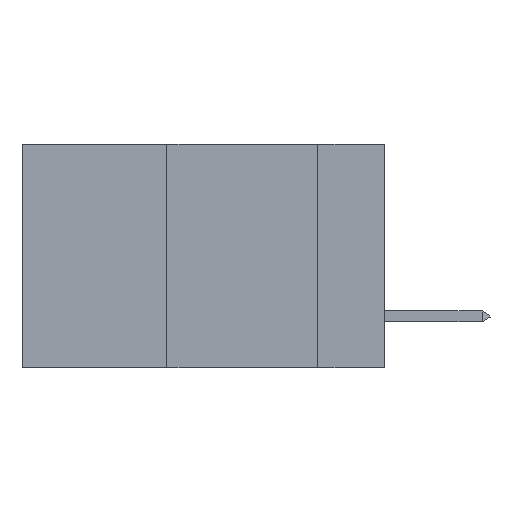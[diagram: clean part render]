
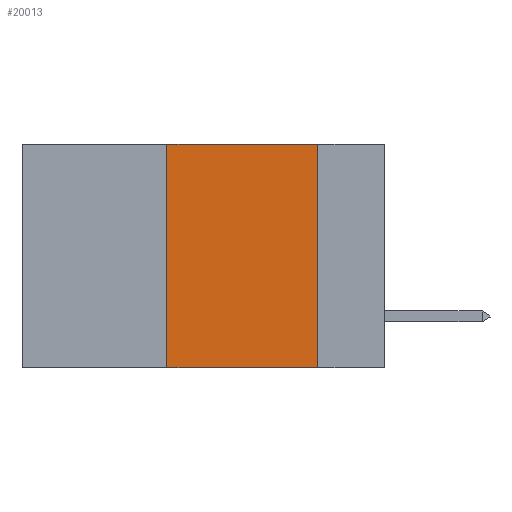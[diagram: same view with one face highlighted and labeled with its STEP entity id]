
A CAD part, left-side view. The second image highlights one B-rep face of the part: STEP entity #20013.
In plain terms, the highlighted planar face has unit normal (-1, 0, 0).
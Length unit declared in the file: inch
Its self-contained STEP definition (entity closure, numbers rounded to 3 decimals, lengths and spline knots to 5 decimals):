
#1392 = ORIENTED_EDGE ( 'NONE', *, *, #19337, .F. ) ;
#1839 = PLANE ( 'NONE',  #29343 ) ;
#2061 = EDGE_CURVE ( 'NONE', #27408, #23974, #2256, .T. ) ;
#2256 = LINE ( 'NONE', #31795, #14855 ) ;
#4063 = EDGE_LOOP ( 'NONE', ( #1392, #5840, #32212, #18051 ) ) ;
#5086 = CARTESIAN_POINT ( 'NONE',  ( 0., 0.6, 0. ) ) ;
#5359 = CARTESIAN_POINT ( 'NONE',  ( 0., 0.6, -0.37 ) ) ;
#5759 = CARTESIAN_POINT ( 'NONE',  ( 0., 0.11, -0.37 ) ) ;
#5840 = ORIENTED_EDGE ( 'NONE', *, *, #32255, .F. ) ;
#8533 = DIRECTION ( 'NONE',  ( 0., 0., -1. ) ) ;
#11196 = DIRECTION ( 'NONE',  ( 0., -1., 0. ) ) ;
#12754 = VERTEX_POINT ( 'NONE', #5759 ) ;
#13351 = VERTEX_POINT ( 'NONE', #32828 ) ;
#14855 = VECTOR ( 'NONE', #38275, 39.37008 ) ;
#16982 = VECTOR ( 'NONE', #25563, 39.37008 ) ;
#18051 = ORIENTED_EDGE ( 'NONE', *, *, #37417, .T. ) ;
#19145 = DIRECTION ( 'NONE',  ( 1., 0., 0. ) ) ;
#19337 = EDGE_CURVE ( 'NONE', #13351, #12754, #20806, .T. ) ;
#20013 = ADVANCED_FACE ( 'NONE', ( #30388 ), #1839, .F. ) ;
#20779 = LINE ( 'NONE', #5359, #36515 ) ;
#20806 = LINE ( 'NONE', #23416, #35171 ) ;
#21681 = CARTESIAN_POINT ( 'NONE',  ( 0., 0.36, -0.37 ) ) ;
#23416 = CARTESIAN_POINT ( 'NONE',  ( 0., 0.11, 0. ) ) ;
#23974 = VERTEX_POINT ( 'NONE', #25890 ) ;
#25368 = LINE ( 'NONE', #5086, #16982 ) ;
#25563 = DIRECTION ( 'NONE',  ( 0., -1., 0. ) ) ;
#25732 = DIRECTION ( 'NONE',  ( 0., 0., -1. ) ) ;
#25890 = CARTESIAN_POINT ( 'NONE',  ( 0., 0.36, 0. ) ) ;
#27408 = VERTEX_POINT ( 'NONE', #21681 ) ;
#28387 = CARTESIAN_POINT ( 'NONE',  ( 0., 0.6, 0. ) ) ;
#29343 = AXIS2_PLACEMENT_3D ( 'NONE', #28387, #19145, #25732 ) ;
#30388 = FACE_OUTER_BOUND ( 'NONE', #4063, .T. ) ;
#31795 = CARTESIAN_POINT ( 'NONE',  ( 0., 0.36, 0. ) ) ;
#32212 = ORIENTED_EDGE ( 'NONE', *, *, #2061, .F. ) ;
#32255 = EDGE_CURVE ( 'NONE', #23974, #13351, #25368, .T. ) ;
#32828 = CARTESIAN_POINT ( 'NONE',  ( 0., 0.11, 0. ) ) ;
#35171 = VECTOR ( 'NONE', #8533, 39.37008 ) ;
#36515 = VECTOR ( 'NONE', #11196, 39.37008 ) ;
#37417 = EDGE_CURVE ( 'NONE', #27408, #12754, #20779, .T. ) ;
#38275 = DIRECTION ( 'NONE',  ( 0., 0., 1. ) ) ;
